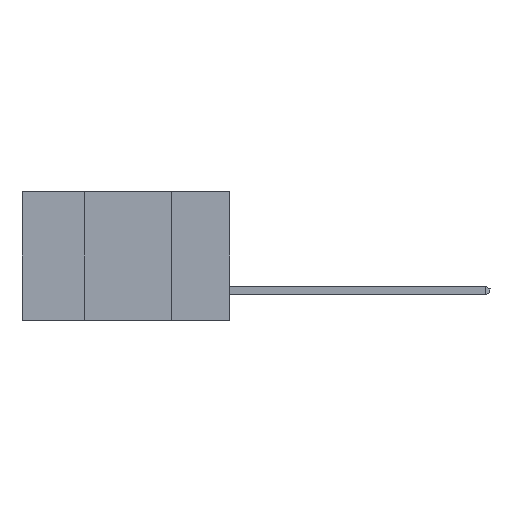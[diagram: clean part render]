
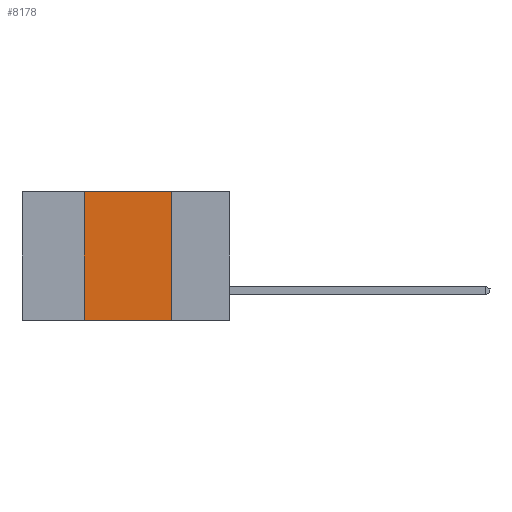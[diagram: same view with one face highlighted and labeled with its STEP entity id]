
A CAD part, left-side view. The second image highlights one B-rep face of the part: STEP entity #8178.
In plain terms, the highlighted planar face has unit normal (-1, 0, 0).
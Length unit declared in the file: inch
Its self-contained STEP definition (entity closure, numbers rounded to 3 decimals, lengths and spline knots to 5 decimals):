
#349 = CARTESIAN_POINT ( 'NONE',  ( 0., 0.6, 0. ) ) ;
#413 = LINE ( 'NONE', #7648, #6920 ) ;
#786 = CARTESIAN_POINT ( 'NONE',  ( 0., 0.42, 0. ) ) ;
#1169 = VERTEX_POINT ( 'NONE', #14263 ) ;
#2774 = DIRECTION ( 'NONE',  ( 0., 0., 1. ) ) ;
#2802 = DIRECTION ( 'NONE',  ( 0., -1., 0. ) ) ;
#3256 = EDGE_CURVE ( 'NONE', #4229, #5062, #4119, .T. ) ;
#4019 = FACE_OUTER_BOUND ( 'NONE', #11516, .T. ) ;
#4119 = LINE ( 'NONE', #8960, #12025 ) ;
#4229 = VERTEX_POINT ( 'NONE', #786 ) ;
#4633 = ORIENTED_EDGE ( 'NONE', *, *, #3256, .F. ) ;
#4743 = CARTESIAN_POINT ( 'NONE',  ( 0., 0.17, 0. ) ) ;
#4988 = LINE ( 'NONE', #8480, #6767 ) ;
#5062 = VERTEX_POINT ( 'NONE', #4743 ) ;
#5155 = AXIS2_PLACEMENT_3D ( 'NONE', #349, #11159, #14730 ) ;
#5283 = VECTOR ( 'NONE', #13534, 39.37008 ) ;
#5548 = EDGE_CURVE ( 'NONE', #1169, #4229, #4988, .T. ) ;
#6647 = VERTEX_POINT ( 'NONE', #6771 ) ;
#6767 = VECTOR ( 'NONE', #2774, 39.37008 ) ;
#6771 = CARTESIAN_POINT ( 'NONE',  ( 0., 0.17, -0.37 ) ) ;
#6920 = VECTOR ( 'NONE', #2802, 39.37008 ) ;
#7615 = DIRECTION ( 'NONE',  ( 0., -1., 0. ) ) ;
#7648 = CARTESIAN_POINT ( 'NONE',  ( 0., 0.6, -0.37 ) ) ;
#7739 = CARTESIAN_POINT ( 'NONE',  ( 0., 0.17, -0.37 ) ) ;
#8178 = ADVANCED_FACE ( 'NONE', ( #4019 ), #11236, .F. ) ;
#8179 = ORIENTED_EDGE ( 'NONE', *, *, #8566, .T. ) ;
#8480 = CARTESIAN_POINT ( 'NONE',  ( 0., 0.42, -0.37 ) ) ;
#8566 = EDGE_CURVE ( 'NONE', #1169, #6647, #413, .T. ) ;
#8960 = CARTESIAN_POINT ( 'NONE',  ( 0., 0.6, 0. ) ) ;
#10739 = ORIENTED_EDGE ( 'NONE', *, *, #5548, .F. ) ;
#11159 = DIRECTION ( 'NONE',  ( 1., 0., 0. ) ) ;
#11236 = PLANE ( 'NONE',  #5155 ) ;
#11516 = EDGE_LOOP ( 'NONE', ( #14474, #4633, #10739, #8179 ) ) ;
#12025 = VECTOR ( 'NONE', #7615, 39.37008 ) ;
#13534 = DIRECTION ( 'NONE',  ( 0., 0., -1. ) ) ;
#13619 = LINE ( 'NONE', #7739, #5283 ) ;
#14263 = CARTESIAN_POINT ( 'NONE',  ( 0., 0.42, -0.37 ) ) ;
#14317 = EDGE_CURVE ( 'NONE', #5062, #6647, #13619, .T. ) ;
#14474 = ORIENTED_EDGE ( 'NONE', *, *, #14317, .F. ) ;
#14730 = DIRECTION ( 'NONE',  ( 0., 0., -1. ) ) ;
